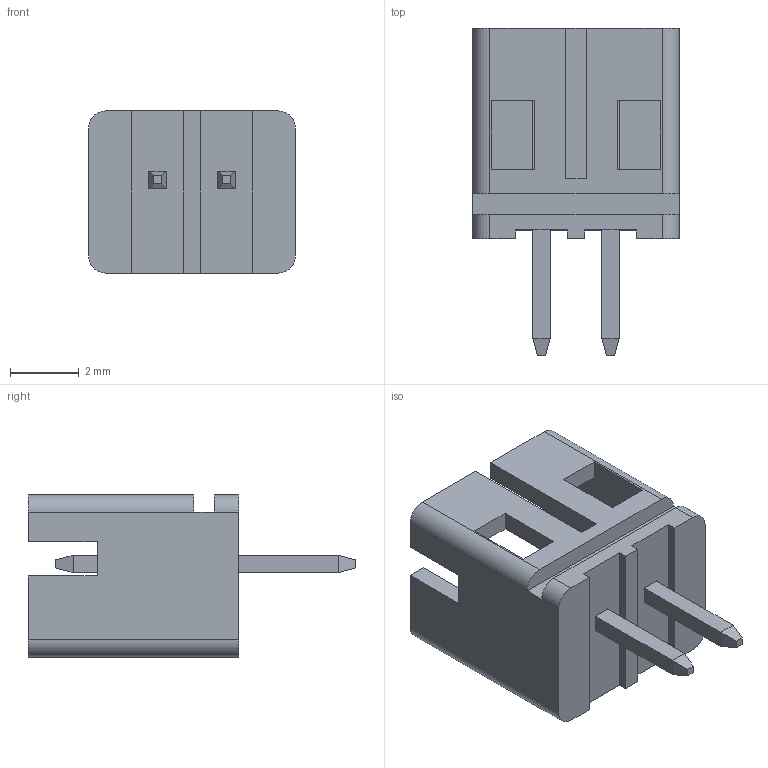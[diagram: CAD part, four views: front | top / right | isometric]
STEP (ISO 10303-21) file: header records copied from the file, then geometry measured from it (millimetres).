
FILE_DESCRIPTION (( 'STEP AP203' ), '1' );
FILE_NAME ('140-502-415-101.STEP', '2020-09-25T11:15:45', ( '' ), ( '' ), 'SwSTEP 2.0', 'SolidWorks 2020', '' );
FILE_SCHEMA (( 'CONFIG_CONTROL_DESIGN' ));
Length unit declared in the file: millimetre
Products named in the file (3): 140-502-415-101; V LI Housing_502; V LI Contact_Str
Assembly tree (3 placements, depth 2):
  140-502-415-101
    V LI Housing_502
    V LI Contact_Str  x2
Bounding box: 6 x 9.5 x 4.7 mm (x, y, z)
Volume: 81.5 mm3; surface area: 302.8 mm2
Topology: 3 solids, 3 shells, 84 faces, 220 edges, 140 vertices
Faces by surface type: plane 78, cylinder 6
Entity records: 2525 total; most frequent: CARTESIAN_POINT 392, ORIENTED_EDGE 384, DIRECTION 356, EDGE_CURVE 192, LINE 180, VECTOR 180, VERTEX_POINT 124, AXIS2_PLACEMENT_3D 88
